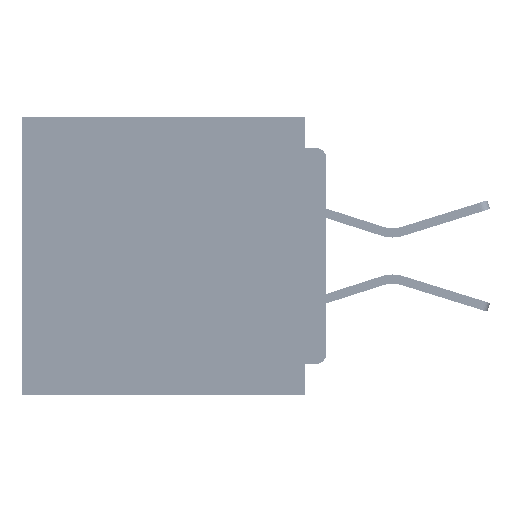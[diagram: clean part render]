
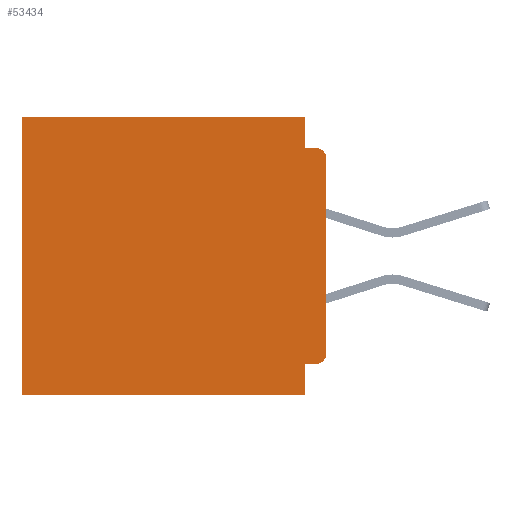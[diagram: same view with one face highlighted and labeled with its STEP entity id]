
A CAD part, left-side view. The second image highlights one B-rep face of the part: STEP entity #53434.
In plain terms, the highlighted planar face has unit normal (-1, 0, 0).
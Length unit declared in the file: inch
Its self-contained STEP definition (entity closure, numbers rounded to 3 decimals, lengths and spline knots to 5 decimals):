
#177 = DIRECTION ( 'NONE',  ( 0., 0., -1. ) ) ;
#1970 = LINE ( 'NONE', #42840, #52882 ) ;
#2300 = AXIS2_PLACEMENT_3D ( 'NONE', #40993, #30656, #67230 ) ;
#2634 = ORIENTED_EDGE ( 'NONE', *, *, #29267, .T. ) ;
#2693 = CARTESIAN_POINT ( 'NONE',  ( 0.3, 0.015, -0.045 ) ) ;
#4574 = EDGE_LOOP ( 'NONE', ( #19157, #2634, #37390, #4790, #54116, #26110, #63046, #9388, #41957, #40994 ) ) ;
#4675 = CIRCLE ( 'NONE', #8258, 0.015 ) ;
#4790 = ORIENTED_EDGE ( 'NONE', *, *, #16412, .F. ) ;
#6039 = CARTESIAN_POINT ( 'NONE',  ( 0.3, 0.031, -0.4 ) ) ;
#6613 = VERTEX_POINT ( 'NONE', #61558 ) ;
#6898 = LINE ( 'NONE', #32200, #33147 ) ;
#7515 = DIRECTION ( 'NONE',  ( -1., 0., 0. ) ) ;
#8258 = AXIS2_PLACEMENT_3D ( 'NONE', #38934, #7515, #44197 ) ;
#9388 = ORIENTED_EDGE ( 'NONE', *, *, #42933, .F. ) ;
#10536 = CARTESIAN_POINT ( 'NONE',  ( 0.3, 0.031, -0.045 ) ) ;
#10757 = VECTOR ( 'NONE', #46072, 39.37008 ) ;
#12071 = LINE ( 'NONE', #12639, #39969 ) ;
#12639 = CARTESIAN_POINT ( 'NONE',  ( 0.3, 0., -0.355 ) ) ;
#14971 = CARTESIAN_POINT ( 'NONE',  ( 0.3, 0.031, -0.355 ) ) ;
#16412 = EDGE_CURVE ( 'NONE', #6613, #53057, #17153, .T. ) ;
#17153 = LINE ( 'NONE', #58475, #29454 ) ;
#17638 = EDGE_CURVE ( 'NONE', #6613, #18150, #6898, .T. ) ;
#18150 = VERTEX_POINT ( 'NONE', #41778 ) ;
#19157 = ORIENTED_EDGE ( 'NONE', *, *, #43812, .F. ) ;
#19771 = VECTOR ( 'NONE', #177, 39.37008 ) ;
#20273 = VERTEX_POINT ( 'NONE', #34522 ) ;
#21985 = AXIS2_PLACEMENT_3D ( 'NONE', #61854, #30557, #67120 ) ;
#23017 = VERTEX_POINT ( 'NONE', #60158 ) ;
#23363 = LINE ( 'NONE', #40345, #65057 ) ;
#23936 = VERTEX_POINT ( 'NONE', #31022 ) ;
#26110 = ORIENTED_EDGE ( 'NONE', *, *, #56970, .T. ) ;
#29267 = EDGE_CURVE ( 'NONE', #23017, #36956, #34461, .T. ) ;
#29454 = VECTOR ( 'NONE', #53032, 39.37008 ) ;
#30115 = EDGE_CURVE ( 'NONE', #48304, #44022, #1970, .T. ) ;
#30557 = DIRECTION ( 'NONE',  ( -1., 0., 0. ) ) ;
#30656 = DIRECTION ( 'NONE',  ( 1., 0., 0. ) ) ;
#30823 = FACE_OUTER_BOUND ( 'NONE', #4574, .T. ) ;
#31022 = CARTESIAN_POINT ( 'NONE',  ( 0.3, 0., -0.34 ) ) ;
#32200 = CARTESIAN_POINT ( 'NONE',  ( 0.3, 0., 0. ) ) ;
#33147 = VECTOR ( 'NONE', #63490, 39.37008 ) ;
#33717 = LINE ( 'NONE', #47245, #19771 ) ;
#34461 = CIRCLE ( 'NONE', #21985, 0.015 ) ;
#34522 = CARTESIAN_POINT ( 'NONE',  ( 0.3, 0.015, -0.355 ) ) ;
#36516 = VERTEX_POINT ( 'NONE', #14971 ) ;
#36956 = VERTEX_POINT ( 'NONE', #2693 ) ;
#37390 = ORIENTED_EDGE ( 'NONE', *, *, #38824, .F. ) ;
#37452 = DIRECTION ( 'NONE',  ( 0., 0., -1. ) ) ;
#38824 = EDGE_CURVE ( 'NONE', #53057, #36956, #52610, .T. ) ;
#38934 = CARTESIAN_POINT ( 'NONE',  ( 0.3, 0.015, -0.34 ) ) ;
#39969 = VECTOR ( 'NONE', #49772, 39.37008 ) ;
#40345 = CARTESIAN_POINT ( 'NONE',  ( 0.3, 0., -0.4 ) ) ;
#40993 = CARTESIAN_POINT ( 'NONE',  ( 0.3, 0., -0.4 ) ) ;
#40994 = ORIENTED_EDGE ( 'NONE', *, *, #48064, .T. ) ;
#41778 = CARTESIAN_POINT ( 'NONE',  ( 0.3, 0.437, 0. ) ) ;
#41957 = ORIENTED_EDGE ( 'NONE', *, *, #52692, .F. ) ;
#42157 = CARTESIAN_POINT ( 'NONE',  ( 0.3, 0.437, -0.4 ) ) ;
#42840 = CARTESIAN_POINT ( 'NONE',  ( 0.3, 0., -0.4 ) ) ;
#42933 = EDGE_CURVE ( 'NONE', #36516, #48304, #64275, .T. ) ;
#43812 = EDGE_CURVE ( 'NONE', #23017, #23936, #23363, .T. ) ;
#44022 = VERTEX_POINT ( 'NONE', #42157 ) ;
#44197 = DIRECTION ( 'NONE',  ( 0., 0., -1. ) ) ;
#44436 = DIRECTION ( 'NONE',  ( 0., 0., -1. ) ) ;
#46009 = CARTESIAN_POINT ( 'NONE',  ( 0.3, 0.031, -0.4 ) ) ;
#46072 = DIRECTION ( 'NONE',  ( 0., -1., 0. ) ) ;
#46237 = PLANE ( 'NONE',  #2300 ) ;
#47245 = CARTESIAN_POINT ( 'NONE',  ( 0.3, 0.437, -0.4 ) ) ;
#48064 = EDGE_CURVE ( 'NONE', #20273, #23936, #4675, .T. ) ;
#48106 = DIRECTION ( 'NONE',  ( 0., 1., 0. ) ) ;
#48304 = VERTEX_POINT ( 'NONE', #46009 ) ;
#49772 = DIRECTION ( 'NONE',  ( 0., 1., 0. ) ) ;
#52126 = VECTOR ( 'NONE', #37452, 39.37008 ) ;
#52610 = LINE ( 'NONE', #67059, #10757 ) ;
#52692 = EDGE_CURVE ( 'NONE', #20273, #36516, #12071, .T. ) ;
#52882 = VECTOR ( 'NONE', #48106, 39.37008 ) ;
#53032 = DIRECTION ( 'NONE',  ( 0., 0., -1. ) ) ;
#53057 = VERTEX_POINT ( 'NONE', #10536 ) ;
#53434 = ADVANCED_FACE ( 'NONE', ( #30823 ), #46237, .F. ) ;
#54116 = ORIENTED_EDGE ( 'NONE', *, *, #17638, .T. ) ;
#56970 = EDGE_CURVE ( 'NONE', #18150, #44022, #33717, .T. ) ;
#58475 = CARTESIAN_POINT ( 'NONE',  ( 0.3, 0.031, 0. ) ) ;
#60158 = CARTESIAN_POINT ( 'NONE',  ( 0.3, 0., -0.06 ) ) ;
#61558 = CARTESIAN_POINT ( 'NONE',  ( 0.3, 0.031, 0. ) ) ;
#61854 = CARTESIAN_POINT ( 'NONE',  ( 0.3, 0.015, -0.06 ) ) ;
#63046 = ORIENTED_EDGE ( 'NONE', *, *, #30115, .F. ) ;
#63490 = DIRECTION ( 'NONE',  ( 0., 1., 0. ) ) ;
#64275 = LINE ( 'NONE', #6039, #52126 ) ;
#65057 = VECTOR ( 'NONE', #44436, 39.37008 ) ;
#67059 = CARTESIAN_POINT ( 'NONE',  ( 0.3, 0., -0.045 ) ) ;
#67120 = DIRECTION ( 'NONE',  ( 0., 0., -1. ) ) ;
#67230 = DIRECTION ( 'NONE',  ( 0., 0., -1. ) ) ;
